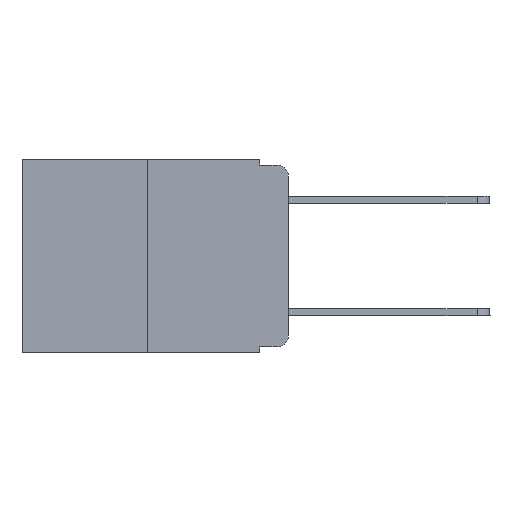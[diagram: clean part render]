
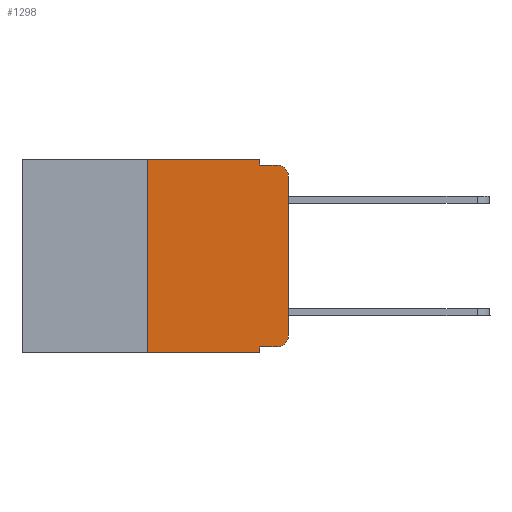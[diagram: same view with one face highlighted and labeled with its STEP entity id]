
A CAD part, left-side view. The second image highlights one B-rep face of the part: STEP entity #1298.
In plain terms, the highlighted planar face has unit normal (-1, 0, 0).
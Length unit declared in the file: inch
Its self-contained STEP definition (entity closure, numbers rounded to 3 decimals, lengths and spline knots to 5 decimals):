
#568 = LINE ( 'NONE', #5645, #7816 ) ;
#625 = CARTESIAN_POINT ( 'NONE',  ( 0., 0.473, -0.343 ) ) ;
#754 = ORIENTED_EDGE ( 'NONE', *, *, #17867, .T. ) ;
#1271 = DIRECTION ( 'NONE',  ( 0., 0., -1. ) ) ;
#1298 = ADVANCED_FACE ( 'NONE', ( #3211 ), #1976, .F. ) ;
#1420 = DIRECTION ( 'NONE',  ( 0., -1., 0. ) ) ;
#1620 = VERTEX_POINT ( 'NONE', #17620 ) ;
#1786 = VERTEX_POINT ( 'NONE', #2417 ) ;
#1976 = PLANE ( 'NONE',  #7370 ) ;
#2179 = VERTEX_POINT ( 'NONE', #5934 ) ;
#2417 = CARTESIAN_POINT ( 'NONE',  ( 0., 0.25, -0.343 ) ) ;
#2495 = CARTESIAN_POINT ( 'NONE',  ( 0., 0.051, 0. ) ) ;
#2571 = CARTESIAN_POINT ( 'NONE',  ( 0., 0., 0. ) ) ;
#3152 = LINE ( 'NONE', #13957, #3587 ) ;
#3193 = VERTEX_POINT ( 'NONE', #15125 ) ;
#3211 = FACE_OUTER_BOUND ( 'NONE', #7733, .T. ) ;
#3254 = LINE ( 'NONE', #4050, #8085 ) ;
#3525 = VECTOR ( 'NONE', #8052, 39.37008 ) ;
#3587 = VECTOR ( 'NONE', #8233, 39.37008 ) ;
#3794 = CIRCLE ( 'NONE', #7219, 0.02 ) ;
#4050 = CARTESIAN_POINT ( 'NONE',  ( 0., 0.25, 0. ) ) ;
#4173 = CARTESIAN_POINT ( 'NONE',  ( 0., 0.051, -0.343 ) ) ;
#4404 = AXIS2_PLACEMENT_3D ( 'NONE', #11030, #6738, #1271 ) ;
#5004 = ORIENTED_EDGE ( 'NONE', *, *, #16975, .F. ) ;
#5085 = DIRECTION ( 'NONE',  ( 0., -1., 0. ) ) ;
#5314 = EDGE_CURVE ( 'NONE', #3193, #10332, #10531, .T. ) ;
#5375 = VECTOR ( 'NONE', #5085, 39.37008 ) ;
#5467 = ORIENTED_EDGE ( 'NONE', *, *, #15495, .T. ) ;
#5506 = VERTEX_POINT ( 'NONE', #17002 ) ;
#5632 = CARTESIAN_POINT ( 'NONE',  ( 0., 0.051, -0.333 ) ) ;
#5645 = CARTESIAN_POINT ( 'NONE',  ( 0., 0.473, 0. ) ) ;
#5850 = VECTOR ( 'NONE', #17955, 39.37008 ) ;
#5931 = ORIENTED_EDGE ( 'NONE', *, *, #17569, .T. ) ;
#5934 = CARTESIAN_POINT ( 'NONE',  ( 0., 0., -0.03 ) ) ;
#6257 = EDGE_CURVE ( 'NONE', #1786, #8344, #16211, .T. ) ;
#6316 = VECTOR ( 'NONE', #16957, 39.37008 ) ;
#6445 = DIRECTION ( 'NONE',  ( 0., -1., 0. ) ) ;
#6738 = DIRECTION ( 'NONE',  ( -1., 0., 0. ) ) ;
#7040 = DIRECTION ( 'NONE',  ( 0., 0., 1. ) ) ;
#7140 = EDGE_CURVE ( 'NONE', #5506, #2179, #17500, .T. ) ;
#7219 = AXIS2_PLACEMENT_3D ( 'NONE', #13473, #11203, #9857 ) ;
#7370 = AXIS2_PLACEMENT_3D ( 'NONE', #17254, #10199, #13146 ) ;
#7619 = ORIENTED_EDGE ( 'NONE', *, *, #7140, .T. ) ;
#7688 = VERTEX_POINT ( 'NONE', #13389 ) ;
#7733 = EDGE_LOOP ( 'NONE', ( #7619, #5931, #17777, #10477, #9689, #13074, #9028, #5004, #5467, #754 ) ) ;
#7798 = CARTESIAN_POINT ( 'NONE',  ( 0., 0.051, -0.01 ) ) ;
#7816 = VECTOR ( 'NONE', #1420, 39.37008 ) ;
#8052 = DIRECTION ( 'NONE',  ( 0., 0., -1. ) ) ;
#8085 = VECTOR ( 'NONE', #7040, 39.37008 ) ;
#8233 = DIRECTION ( 'NONE',  ( 0., 0., -1. ) ) ;
#8344 = VERTEX_POINT ( 'NONE', #4173 ) ;
#8525 = VECTOR ( 'NONE', #6445, 39.37008 ) ;
#8767 = CARTESIAN_POINT ( 'NONE',  ( 0., 0.051, -0.01 ) ) ;
#9028 = ORIENTED_EDGE ( 'NONE', *, *, #6257, .T. ) ;
#9119 = VERTEX_POINT ( 'NONE', #5632 ) ;
#9520 = VERTEX_POINT ( 'NONE', #13490 ) ;
#9573 = LINE ( 'NONE', #17688, #5375 ) ;
#9689 = ORIENTED_EDGE ( 'NONE', *, *, #15025, .F. ) ;
#9857 = DIRECTION ( 'NONE',  ( 0., 0., -1. ) ) ;
#10199 = DIRECTION ( 'NONE',  ( 1., 0., 0. ) ) ;
#10332 = VERTEX_POINT ( 'NONE', #8767 ) ;
#10477 = ORIENTED_EDGE ( 'NONE', *, *, #5314, .F. ) ;
#10531 = LINE ( 'NONE', #2495, #3525 ) ;
#11030 = CARTESIAN_POINT ( 'NONE',  ( 0., 0.02, -0.313 ) ) ;
#11203 = DIRECTION ( 'NONE',  ( -1., 0., 0. ) ) ;
#12431 = EDGE_CURVE ( 'NONE', #10332, #1620, #14692, .T. ) ;
#13074 = ORIENTED_EDGE ( 'NONE', *, *, #13301, .F. ) ;
#13146 = DIRECTION ( 'NONE',  ( 0., 0., -1. ) ) ;
#13301 = EDGE_CURVE ( 'NONE', #1786, #7688, #3254, .T. ) ;
#13389 = CARTESIAN_POINT ( 'NONE',  ( 0., 0.25, 0. ) ) ;
#13473 = CARTESIAN_POINT ( 'NONE',  ( 0., 0.02, -0.03 ) ) ;
#13490 = CARTESIAN_POINT ( 'NONE',  ( 0., 0.02, -0.333 ) ) ;
#13957 = CARTESIAN_POINT ( 'NONE',  ( 0., 0.051, 0. ) ) ;
#14102 = CIRCLE ( 'NONE', #4404, 0.02 ) ;
#14692 = LINE ( 'NONE', #7798, #8525 ) ;
#15025 = EDGE_CURVE ( 'NONE', #7688, #3193, #568, .T. ) ;
#15125 = CARTESIAN_POINT ( 'NONE',  ( 0., 0.051, 0. ) ) ;
#15495 = EDGE_CURVE ( 'NONE', #9119, #9520, #9573, .T. ) ;
#16211 = LINE ( 'NONE', #625, #6316 ) ;
#16957 = DIRECTION ( 'NONE',  ( 0., -1., 0. ) ) ;
#16975 = EDGE_CURVE ( 'NONE', #9119, #8344, #3152, .T. ) ;
#17002 = CARTESIAN_POINT ( 'NONE',  ( 0., 0., -0.313 ) ) ;
#17254 = CARTESIAN_POINT ( 'NONE',  ( 0., 0.473, 0. ) ) ;
#17500 = LINE ( 'NONE', #2571, #5850 ) ;
#17569 = EDGE_CURVE ( 'NONE', #2179, #1620, #3794, .T. ) ;
#17620 = CARTESIAN_POINT ( 'NONE',  ( 0., 0.02, -0.01 ) ) ;
#17688 = CARTESIAN_POINT ( 'NONE',  ( 0., 0.051, -0.333 ) ) ;
#17777 = ORIENTED_EDGE ( 'NONE', *, *, #12431, .F. ) ;
#17867 = EDGE_CURVE ( 'NONE', #9520, #5506, #14102, .T. ) ;
#17955 = DIRECTION ( 'NONE',  ( 0., 0., 1. ) ) ;
